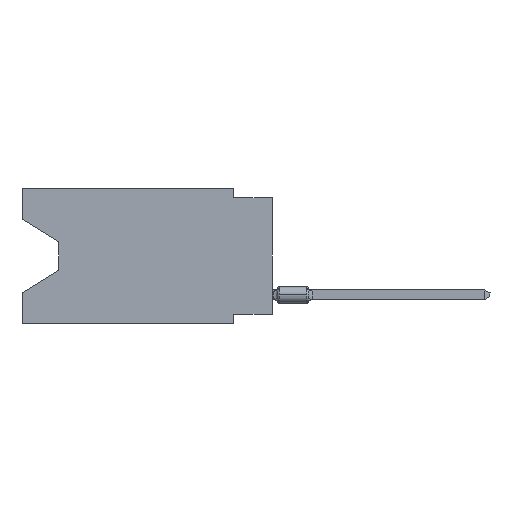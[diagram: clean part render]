
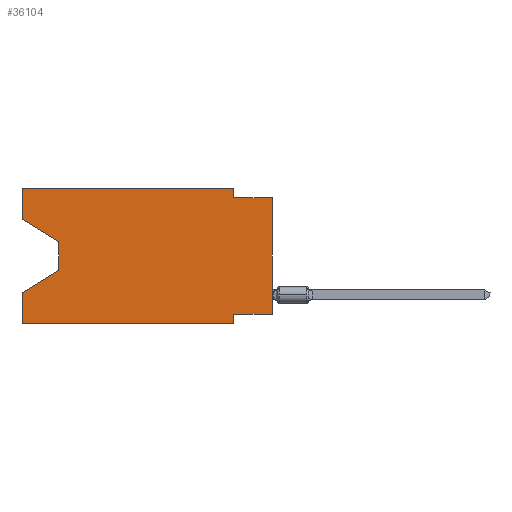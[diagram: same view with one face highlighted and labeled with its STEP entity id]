
A CAD part, left-side view. The second image highlights one B-rep face of the part: STEP entity #36104.
In plain terms, the highlighted planar face has unit normal (-1, 0, 0).
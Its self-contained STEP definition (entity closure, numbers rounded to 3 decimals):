
#1871 = DIRECTION ( 'NONE',  ( 1., 0., 0. ) ) ;
#4146 = ORIENTED_EDGE ( 'NONE', *, *, #24419, .T. ) ;
#5331 = CARTESIAN_POINT ( 'NONE',  ( 0., 0., 0. ) ) ;
#7298 = DIRECTION ( 'NONE',  ( 0., 0.855, -0.519 ) ) ;
#7941 = VECTOR ( 'NONE', #37489, 1000. ) ;
#9243 = DIRECTION ( 'NONE',  ( 0., 0., -1. ) ) ;
#10327 = VECTOR ( 'NONE', #75680, 1000. ) ;
#11277 = VECTOR ( 'NONE', #93438, 1000. ) ;
#15034 = LINE ( 'NONE', #108836, #75059 ) ;
#17729 = FACE_OUTER_BOUND ( 'NONE', #87136, .T. ) ;
#17847 = VERTEX_POINT ( 'NONE', #41791 ) ;
#18965 = VECTOR ( 'NONE', #67121, 1000. ) ;
#19230 = VECTOR ( 'NONE', #79818, 1000. ) ;
#19925 = PLANE ( 'NONE',  #37028 ) ;
#22347 = ORIENTED_EDGE ( 'NONE', *, *, #85073, .T. ) ;
#23188 = VERTEX_POINT ( 'NONE', #47443 ) ;
#23315 = EDGE_CURVE ( 'NONE', #44879, #70710, #68865, .T. ) ;
#24264 = CARTESIAN_POINT ( 'NONE',  ( 0., 13.97, -5.385 ) ) ;
#24419 = EDGE_CURVE ( 'NONE', #95099, #23188, #60391, .T. ) ;
#24914 = CARTESIAN_POINT ( 'NONE',  ( 0., 16.383, 0. ) ) ;
#26349 = LINE ( 'NONE', #77777, #83784 ) ;
#28482 = CARTESIAN_POINT ( 'NONE',  ( 0., 16.383, -2.038 ) ) ;
#28531 = LINE ( 'NONE', #30733, #107790 ) ;
#30733 = CARTESIAN_POINT ( 'NONE',  ( 0., 13.97, -3.505 ) ) ;
#31333 = DIRECTION ( 'NONE',  ( 0., 0., 1. ) ) ;
#31418 = ORIENTED_EDGE ( 'NONE', *, *, #52333, .T. ) ;
#32643 = LINE ( 'NONE', #105327, #18965 ) ;
#33653 = ORIENTED_EDGE ( 'NONE', *, *, #88674, .F. ) ;
#34298 = VERTEX_POINT ( 'NONE', #91916 ) ;
#35059 = VECTOR ( 'NONE', #31333, 1000. ) ;
#35395 = DIRECTION ( 'NONE',  ( 0., 1., 0. ) ) ;
#36104 = ADVANCED_FACE ( 'NONE', ( #17729 ), #19925, .F. ) ;
#36507 = CARTESIAN_POINT ( 'NONE',  ( 0., 13.97, -3.505 ) ) ;
#37028 = AXIS2_PLACEMENT_3D ( 'NONE', #95692, #1871, #9243 ) ;
#37489 = DIRECTION ( 'NONE',  ( 0., -1., 0. ) ) ;
#39489 = CARTESIAN_POINT ( 'NONE',  ( 0., 16.383, 0. ) ) ;
#40197 = ORIENTED_EDGE ( 'NONE', *, *, #89355, .F. ) ;
#40534 = DIRECTION ( 'NONE',  ( 0., 0., -1. ) ) ;
#41456 = LINE ( 'NONE', #58933, #11277 ) ;
#41791 = CARTESIAN_POINT ( 'NONE',  ( 0., 0., -0.635 ) ) ;
#44879 = VERTEX_POINT ( 'NONE', #28482 ) ;
#45165 = VERTEX_POINT ( 'NONE', #102421 ) ;
#46464 = CARTESIAN_POINT ( 'NONE',  ( 0., 0., -0.635 ) ) ;
#46515 = CARTESIAN_POINT ( 'NONE',  ( 0., 2.54, 0. ) ) ;
#46520 = LINE ( 'NONE', #73063, #7941 ) ;
#47443 = CARTESIAN_POINT ( 'NONE',  ( 0., 16.383, -6.852 ) ) ;
#47890 = CARTESIAN_POINT ( 'NONE',  ( 0., 2.54, -8.89 ) ) ;
#48999 = LINE ( 'NONE', #47890, #64411 ) ;
#49914 = EDGE_CURVE ( 'NONE', #44879, #104368, #67309, .T. ) ;
#52333 = EDGE_CURVE ( 'NONE', #34298, #45165, #41456, .T. ) ;
#57115 = ORIENTED_EDGE ( 'NONE', *, *, #86469, .F. ) ;
#58484 = ORIENTED_EDGE ( 'NONE', *, *, #67896, .F. ) ;
#58933 = CARTESIAN_POINT ( 'NONE',  ( 0., 16.383, -8.89 ) ) ;
#60248 = CARTESIAN_POINT ( 'NONE',  ( 0., 0., -8.255 ) ) ;
#60391 = LINE ( 'NONE', #24264, #97200 ) ;
#64411 = VECTOR ( 'NONE', #40534, 1000. ) ;
#65096 = CARTESIAN_POINT ( 'NONE',  ( 0., 2.54, -8.255 ) ) ;
#65223 = DIRECTION ( 'NONE',  ( 0., 0., -1. ) ) ;
#65679 = ORIENTED_EDGE ( 'NONE', *, *, #84840, .F. ) ;
#67020 = DIRECTION ( 'NONE',  ( 0., 0., -1. ) ) ;
#67121 = DIRECTION ( 'NONE',  ( 0., 0., 1. ) ) ;
#67309 = LINE ( 'NONE', #24914, #110125 ) ;
#67896 = EDGE_CURVE ( 'NONE', #108401, #45165, #48999, .T. ) ;
#68865 = LINE ( 'NONE', #103325, #10327 ) ;
#70513 = VERTEX_POINT ( 'NONE', #60248 ) ;
#70710 = VERTEX_POINT ( 'NONE', #36507 ) ;
#73063 = CARTESIAN_POINT ( 'NONE',  ( 0., 16.383, 0. ) ) ;
#75059 = VECTOR ( 'NONE', #67020, 1000. ) ;
#75680 = DIRECTION ( 'NONE',  ( 0., -0.855, -0.519 ) ) ;
#75732 = ORIENTED_EDGE ( 'NONE', *, *, #101557, .F. ) ;
#77164 = VERTEX_POINT ( 'NONE', #46515 ) ;
#77777 = CARTESIAN_POINT ( 'NONE',  ( 0., 0., -8.255 ) ) ;
#79818 = DIRECTION ( 'NONE',  ( 0., -1., 0. ) ) ;
#83145 = DIRECTION ( 'NONE',  ( 0., 0., 1. ) ) ;
#83784 = VECTOR ( 'NONE', #35395, 1000. ) ;
#84840 = EDGE_CURVE ( 'NONE', #70513, #108401, #26349, .T. ) ;
#85073 = EDGE_CURVE ( 'NONE', #70513, #17847, #93504, .T. ) ;
#86469 = EDGE_CURVE ( 'NONE', #104368, #77164, #46520, .T. ) ;
#87136 = EDGE_LOOP ( 'NONE', ( #104580, #103261, #4146, #75732, #31418, #58484, #65679, #22347, #40197, #33653, #57115, #89941 ) ) ;
#88674 = EDGE_CURVE ( 'NONE', #77164, #95350, #15034, .T. ) ;
#89355 = EDGE_CURVE ( 'NONE', #95350, #17847, #107457, .T. ) ;
#89941 = ORIENTED_EDGE ( 'NONE', *, *, #49914, .F. ) ;
#90176 = EDGE_CURVE ( 'NONE', #70710, #95099, #28531, .T. ) ;
#90375 = CARTESIAN_POINT ( 'NONE',  ( 0., 13.97, -5.385 ) ) ;
#91916 = CARTESIAN_POINT ( 'NONE',  ( 0., 16.383, -8.89 ) ) ;
#93438 = DIRECTION ( 'NONE',  ( 0., -1., 0. ) ) ;
#93504 = LINE ( 'NONE', #5331, #35059 ) ;
#95099 = VERTEX_POINT ( 'NONE', #90375 ) ;
#95350 = VERTEX_POINT ( 'NONE', #108988 ) ;
#95692 = CARTESIAN_POINT ( 'NONE',  ( 0., 16.383, 0. ) ) ;
#97200 = VECTOR ( 'NONE', #7298, 1000. ) ;
#101557 = EDGE_CURVE ( 'NONE', #34298, #23188, #32643, .T. ) ;
#102421 = CARTESIAN_POINT ( 'NONE',  ( 0., 2.54, -8.89 ) ) ;
#103261 = ORIENTED_EDGE ( 'NONE', *, *, #90176, .T. ) ;
#103325 = CARTESIAN_POINT ( 'NONE',  ( 0., 16.383, -2.038 ) ) ;
#104368 = VERTEX_POINT ( 'NONE', #39489 ) ;
#104580 = ORIENTED_EDGE ( 'NONE', *, *, #23315, .T. ) ;
#105327 = CARTESIAN_POINT ( 'NONE',  ( 0., 16.383, 0. ) ) ;
#107457 = LINE ( 'NONE', #46464, #19230 ) ;
#107790 = VECTOR ( 'NONE', #65223, 1000. ) ;
#108401 = VERTEX_POINT ( 'NONE', #65096 ) ;
#108836 = CARTESIAN_POINT ( 'NONE',  ( 0., 2.54, 0. ) ) ;
#108988 = CARTESIAN_POINT ( 'NONE',  ( 0., 2.54, -0.635 ) ) ;
#110125 = VECTOR ( 'NONE', #83145, 1000. ) ;
